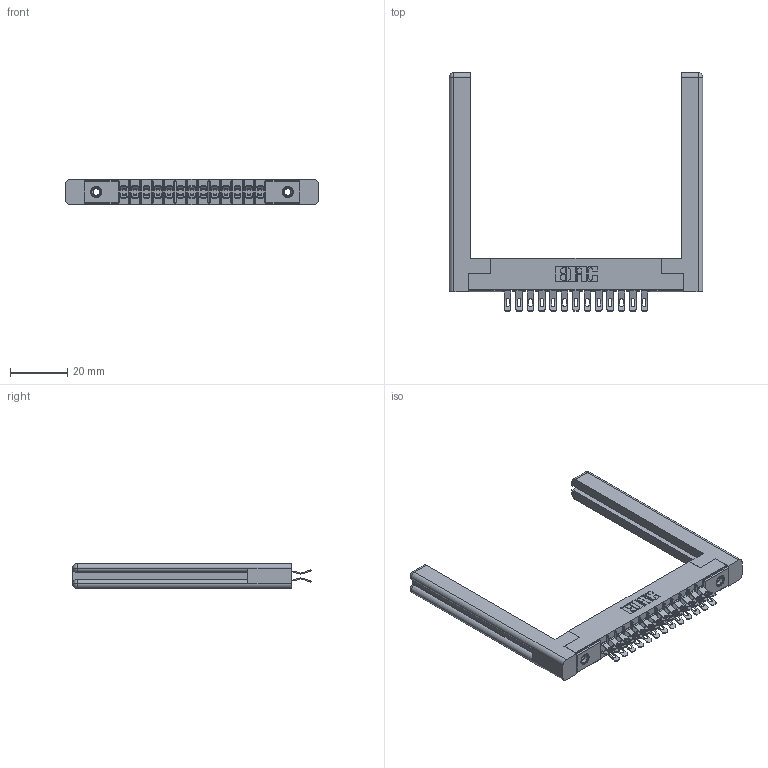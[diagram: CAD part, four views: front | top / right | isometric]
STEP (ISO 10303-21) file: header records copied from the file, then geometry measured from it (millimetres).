
FILE_DESCRIPTION (( 'STEP AP203' ), '1' );
FILE_NAME ('355-026-555-558.STEP', '2019-09-11T05:48:27', ( '' ), ( '' ), 'SwSTEP 2.0', 'SolidWorks 2016', '' );
FILE_SCHEMA (( 'CONFIG_CONTROL_DESIGN' ));
Length unit declared in the file: inch
Products named in the file (5): 345-250-001_345-250-001-102; 305 Part_.156 Dia; 305-290-001_555; 355-026-555-558; 307-220-058
Assembly tree (31 placements, depth 2):
  355-026-555-558
    305 Part_.156 Dia
    305-290-001_555  x26
    345-250-001_345-250-001-102  x2
    307-220-058  x2
Bounding box: 88.14 x 83.06 x 8.71 mm (x, y, z)
Volume: 13155.3 mm3; surface area: 15639.3 mm2
Topology: 31 solids, 31 shells, 1974 faces, 5805 edges, 3786 vertices
Faces by surface type: plane 984, cylinder 914, sphere 52, cone 12, torus 12
Entity records: 20863 total; most frequent: CARTESIAN_POINT 3486, ORIENTED_EDGE 3388, DIRECTION 3352, EDGE_CURVE 1694, LINE 1308, VECTOR 1308, VERTEX_POINT 1086, AXIS2_PLACEMENT_3D 1022
